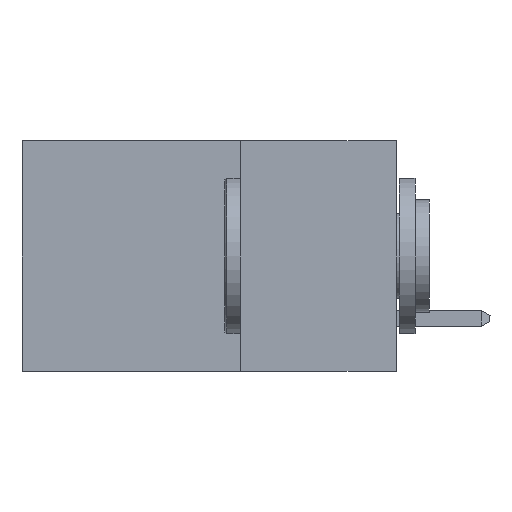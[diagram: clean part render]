
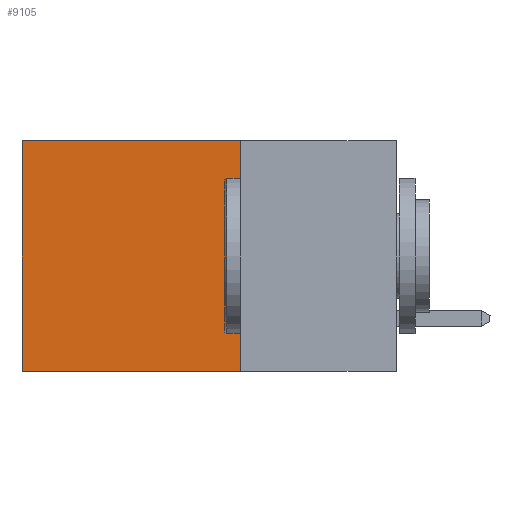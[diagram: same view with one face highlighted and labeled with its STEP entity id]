
A CAD part, left-side view. The second image highlights one B-rep face of the part: STEP entity #9105.
In plain terms, the highlighted planar face has unit normal (-1, 0, 0).
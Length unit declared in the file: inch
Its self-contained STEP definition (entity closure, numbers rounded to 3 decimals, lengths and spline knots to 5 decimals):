
#364 = VERTEX_POINT ( 'NONE', #6541 ) ;
#618 = VERTEX_POINT ( 'NONE', #10362 ) ;
#762 = VERTEX_POINT ( 'NONE', #11846 ) ;
#801 = DIRECTION ( 'NONE',  ( 0., 0., -1. ) ) ;
#951 = VECTOR ( 'NONE', #1304, 39.37008 ) ;
#1276 = PLANE ( 'NONE',  #9256 ) ;
#1304 = DIRECTION ( 'NONE',  ( 0., 0., -1. ) ) ;
#1620 = ORIENTED_EDGE ( 'NONE', *, *, #11473, .F. ) ;
#1787 = CARTESIAN_POINT ( 'NONE',  ( 0.2615, 0.25, 0. ) ) ;
#2454 = CARTESIAN_POINT ( 'NONE',  ( 0.2615, 0.25, -0.37 ) ) ;
#2727 = EDGE_CURVE ( 'NONE', #618, #2808, #4442, .T. ) ;
#2808 = VERTEX_POINT ( 'NONE', #7919 ) ;
#2912 = LINE ( 'NONE', #1787, #8937 ) ;
#3186 = EDGE_CURVE ( 'NONE', #762, #2808, #8234, .T. ) ;
#3192 = EDGE_LOOP ( 'NONE', ( #6807, #12508, #1620, #15661 ) ) ;
#4095 = DIRECTION ( 'NONE',  ( 0., 1., 0. ) ) ;
#4427 = VECTOR ( 'NONE', #4095, 39.37008 ) ;
#4442 = LINE ( 'NONE', #10871, #951 ) ;
#4456 = DIRECTION ( 'NONE',  ( 0., 1., 0. ) ) ;
#4934 = EDGE_CURVE ( 'NONE', #364, #618, #2912, .T. ) ;
#5230 = DIRECTION ( 'NONE',  ( 1., 0., 0. ) ) ;
#6541 = CARTESIAN_POINT ( 'NONE',  ( 0.2615, 0.25, 0. ) ) ;
#6807 = ORIENTED_EDGE ( 'NONE', *, *, #2727, .T. ) ;
#7919 = CARTESIAN_POINT ( 'NONE',  ( 0.2615, 0.6, -0.37 ) ) ;
#8234 = LINE ( 'NONE', #2454, #4427 ) ;
#8937 = VECTOR ( 'NONE', #4456, 39.37008 ) ;
#9105 = ADVANCED_FACE ( 'NONE', ( #13599 ), #1276, .F. ) ;
#9256 = AXIS2_PLACEMENT_3D ( 'NONE', #13865, #5230, #13926 ) ;
#10362 = CARTESIAN_POINT ( 'NONE',  ( 0.2615, 0.6, 0. ) ) ;
#10871 = CARTESIAN_POINT ( 'NONE',  ( 0.2615, 0.6, -0.37 ) ) ;
#11473 = EDGE_CURVE ( 'NONE', #364, #762, #15753, .T. ) ;
#11846 = CARTESIAN_POINT ( 'NONE',  ( 0.2615, 0.25, -0.37 ) ) ;
#12266 = CARTESIAN_POINT ( 'NONE',  ( 0.2615, 0.25, -0.37 ) ) ;
#12508 = ORIENTED_EDGE ( 'NONE', *, *, #3186, .F. ) ;
#13328 = VECTOR ( 'NONE', #801, 39.37008 ) ;
#13599 = FACE_OUTER_BOUND ( 'NONE', #3192, .T. ) ;
#13865 = CARTESIAN_POINT ( 'NONE',  ( 0.2615, 0.25, -0.37 ) ) ;
#13926 = DIRECTION ( 'NONE',  ( 0., 0., -1. ) ) ;
#15661 = ORIENTED_EDGE ( 'NONE', *, *, #4934, .T. ) ;
#15753 = LINE ( 'NONE', #12266, #13328 ) ;
